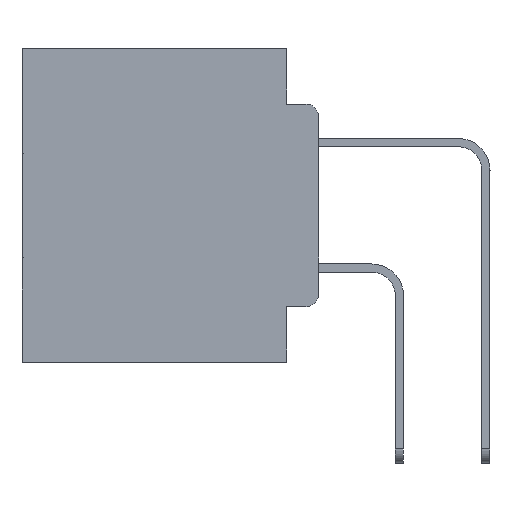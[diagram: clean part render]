
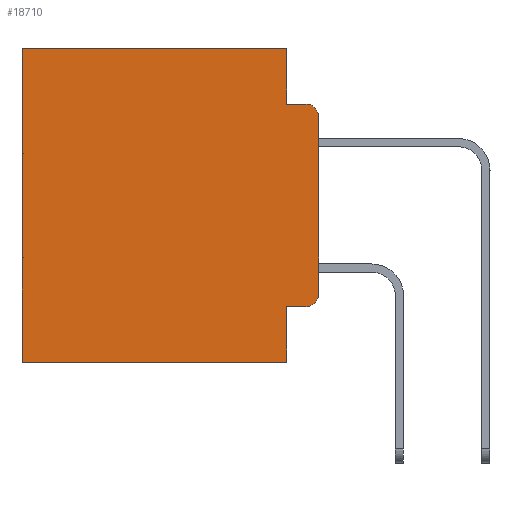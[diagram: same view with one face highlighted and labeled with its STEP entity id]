
A CAD part, left-side view. The second image highlights one B-rep face of the part: STEP entity #18710.
In plain terms, the highlighted planar face has unit normal (-1, 0, 0).
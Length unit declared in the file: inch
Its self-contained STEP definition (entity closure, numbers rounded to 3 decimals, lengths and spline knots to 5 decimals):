
#198 = CARTESIAN_POINT ( 'NONE',  ( 0.298, 0.02, -0.3915 ) ) ;
#665 = EDGE_CURVE ( 'NONE', #22851, #27259, #24477, .T. ) ;
#1310 = CIRCLE ( 'NONE', #31353, 0.02 ) ;
#1446 = DIRECTION ( 'NONE',  ( 0., 0., -1. ) ) ;
#1480 = LINE ( 'NONE', #27513, #29943 ) ;
#1779 = DIRECTION ( 'NONE',  ( 0., 0., -1. ) ) ;
#3497 = DIRECTION ( 'NONE',  ( 0., 1., 0. ) ) ;
#3581 = CARTESIAN_POINT ( 'NONE',  ( 0.298, 0.051, -0.0885 ) ) ;
#4087 = FACE_OUTER_BOUND ( 'NONE', #27165, .T. ) ;
#4252 = DIRECTION ( 'NONE',  ( 1., 0., 0. ) ) ;
#5407 = VERTEX_POINT ( 'NONE', #10093 ) ;
#5845 = LINE ( 'NONE', #8734, #14918 ) ;
#6625 = PLANE ( 'NONE',  #14571 ) ;
#6775 = VECTOR ( 'NONE', #30478, 39.37008 ) ;
#6914 = EDGE_CURVE ( 'NONE', #32842, #27259, #20118, .T. ) ;
#7009 = VECTOR ( 'NONE', #17018, 39.37008 ) ;
#7472 = CARTESIAN_POINT ( 'NONE',  ( 0.298, 0.051, -0.0885 ) ) ;
#7968 = CARTESIAN_POINT ( 'NONE',  ( 0.298, 0., -0.1085 ) ) ;
#8734 = CARTESIAN_POINT ( 'NONE',  ( 0.298, 0.051, 0. ) ) ;
#8881 = EDGE_CURVE ( 'NONE', #22851, #14485, #1310, .T. ) ;
#9212 = DIRECTION ( 'NONE',  ( 0., 1., 0. ) ) ;
#10093 = CARTESIAN_POINT ( 'NONE',  ( 0.298, 0.473, 0. ) ) ;
#10192 = VERTEX_POINT ( 'NONE', #27141 ) ;
#10586 = ORIENTED_EDGE ( 'NONE', *, *, #665, .F. ) ;
#11232 = CARTESIAN_POINT ( 'NONE',  ( 0.298, 0., 0. ) ) ;
#11244 = ORIENTED_EDGE ( 'NONE', *, *, #26009, .T. ) ;
#11377 = EDGE_CURVE ( 'NONE', #27473, #5407, #26826, .T. ) ;
#11404 = CARTESIAN_POINT ( 'NONE',  ( 0.298, 0., 0. ) ) ;
#11587 = ORIENTED_EDGE ( 'NONE', *, *, #25850, .F. ) ;
#11971 = VECTOR ( 'NONE', #1446, 39.37008 ) ;
#12186 = DIRECTION ( 'NONE',  ( 0., 0., -1. ) ) ;
#13470 = VERTEX_POINT ( 'NONE', #21737 ) ;
#13791 = VECTOR ( 'NONE', #21196, 39.37008 ) ;
#14485 = VERTEX_POINT ( 'NONE', #33145 ) ;
#14571 = AXIS2_PLACEMENT_3D ( 'NONE', #32134, #4252, #12186 ) ;
#14888 = CARTESIAN_POINT ( 'NONE',  ( 0.298, 0.02, -0.4115 ) ) ;
#14918 = VECTOR ( 'NONE', #23659, 39.37008 ) ;
#15415 = CARTESIAN_POINT ( 'NONE',  ( 0.298, 0.051, 0. ) ) ;
#16427 = EDGE_CURVE ( 'NONE', #5407, #10192, #27569, .T. ) ;
#16457 = VERTEX_POINT ( 'NONE', #29614 ) ;
#17018 = DIRECTION ( 'NONE',  ( 0., 0., -1. ) ) ;
#17131 = ORIENTED_EDGE ( 'NONE', *, *, #16427, .T. ) ;
#17231 = VERTEX_POINT ( 'NONE', #3581 ) ;
#18540 = VECTOR ( 'NONE', #9212, 39.37008 ) ;
#18710 = ADVANCED_FACE ( 'NONE', ( #4087 ), #6625, .F. ) ;
#19200 = CARTESIAN_POINT ( 'NONE',  ( 0.298, 0.473, 0. ) ) ;
#19717 = ORIENTED_EDGE ( 'NONE', *, *, #22724, .F. ) ;
#20025 = ORIENTED_EDGE ( 'NONE', *, *, #8881, .T. ) ;
#20118 = CIRCLE ( 'NONE', #31890, 0.02 ) ;
#20708 = DIRECTION ( 'NONE',  ( 0., 0., -1. ) ) ;
#21196 = DIRECTION ( 'NONE',  ( 0., 0., -1. ) ) ;
#21737 = CARTESIAN_POINT ( 'NONE',  ( 0.298, 0.051, -0.4115 ) ) ;
#22058 = EDGE_CURVE ( 'NONE', #16457, #10192, #26514, .T. ) ;
#22429 = DIRECTION ( 'NONE',  ( -1., 0., 0. ) ) ;
#22724 = EDGE_CURVE ( 'NONE', #17231, #14485, #33134, .T. ) ;
#22851 = VERTEX_POINT ( 'NONE', #7968 ) ;
#23659 = DIRECTION ( 'NONE',  ( 0., 0., -1. ) ) ;
#24477 = LINE ( 'NONE', #11404, #11971 ) ;
#24650 = EDGE_CURVE ( 'NONE', #13470, #16457, #31596, .T. ) ;
#25287 = CARTESIAN_POINT ( 'NONE',  ( 0.298, 0.02, -0.1085 ) ) ;
#25701 = ORIENTED_EDGE ( 'NONE', *, *, #11377, .T. ) ;
#25842 = ORIENTED_EDGE ( 'NONE', *, *, #6914, .T. ) ;
#25850 = EDGE_CURVE ( 'NONE', #27473, #17231, #5845, .T. ) ;
#26009 = EDGE_CURVE ( 'NONE', #13470, #32842, #1480, .T. ) ;
#26406 = CARTESIAN_POINT ( 'NONE',  ( 0.298, 0.051, 0. ) ) ;
#26514 = LINE ( 'NONE', #29037, #27657 ) ;
#26699 = DIRECTION ( 'NONE',  ( -1., 0., 0. ) ) ;
#26826 = LINE ( 'NONE', #11232, #18540 ) ;
#27141 = CARTESIAN_POINT ( 'NONE',  ( 0.298, 0.473, -0.5 ) ) ;
#27165 = EDGE_LOOP ( 'NONE', ( #10586, #20025, #19717, #11587, #25701, #17131, #29151, #31177, #11244, #25842 ) ) ;
#27259 = VERTEX_POINT ( 'NONE', #29878 ) ;
#27473 = VERTEX_POINT ( 'NONE', #15415 ) ;
#27513 = CARTESIAN_POINT ( 'NONE',  ( 0.298, 0.051, -0.4115 ) ) ;
#27569 = LINE ( 'NONE', #19200, #7009 ) ;
#27657 = VECTOR ( 'NONE', #3497, 39.37008 ) ;
#29037 = CARTESIAN_POINT ( 'NONE',  ( 0.298, 0., -0.5 ) ) ;
#29151 = ORIENTED_EDGE ( 'NONE', *, *, #22058, .F. ) ;
#29614 = CARTESIAN_POINT ( 'NONE',  ( 0.298, 0.051, -0.5 ) ) ;
#29878 = CARTESIAN_POINT ( 'NONE',  ( 0.298, 0., -0.3915 ) ) ;
#29943 = VECTOR ( 'NONE', #32698, 39.37008 ) ;
#30478 = DIRECTION ( 'NONE',  ( 0., -1., 0. ) ) ;
#31177 = ORIENTED_EDGE ( 'NONE', *, *, #24650, .F. ) ;
#31353 = AXIS2_PLACEMENT_3D ( 'NONE', #25287, #22429, #1779 ) ;
#31596 = LINE ( 'NONE', #26406, #13791 ) ;
#31890 = AXIS2_PLACEMENT_3D ( 'NONE', #198, #26699, #20708 ) ;
#32134 = CARTESIAN_POINT ( 'NONE',  ( 0.298, 0., 0. ) ) ;
#32698 = DIRECTION ( 'NONE',  ( 0., -1., 0. ) ) ;
#32842 = VERTEX_POINT ( 'NONE', #14888 ) ;
#33134 = LINE ( 'NONE', #7472, #6775 ) ;
#33145 = CARTESIAN_POINT ( 'NONE',  ( 0.298, 0.02, -0.0885 ) ) ;
